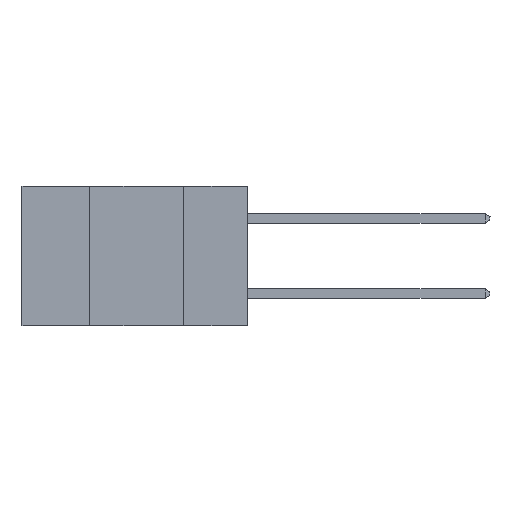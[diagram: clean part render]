
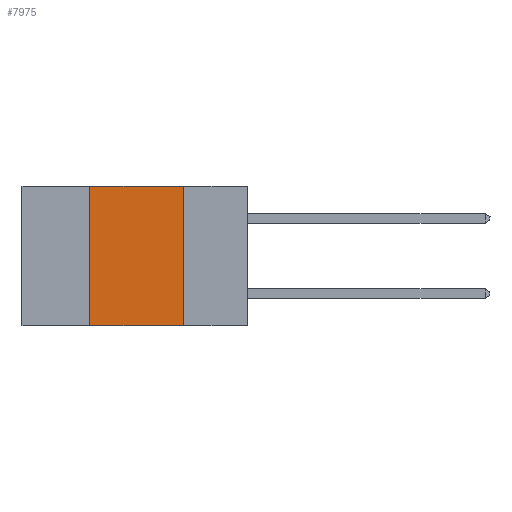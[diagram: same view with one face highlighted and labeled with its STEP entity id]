
A CAD part, left-side view. The second image highlights one B-rep face of the part: STEP entity #7975.
In plain terms, the highlighted planar face has unit normal (-1, 0, 0).
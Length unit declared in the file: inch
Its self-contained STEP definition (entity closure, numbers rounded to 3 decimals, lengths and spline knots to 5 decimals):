
#816 = DIRECTION ( 'NONE',  ( 0., -1., 0. ) ) ;
#1131 = VECTOR ( 'NONE', #14248, 39.37008 ) ;
#1354 = CARTESIAN_POINT ( 'NONE',  ( 0., 0.17, 0. ) ) ;
#2077 = AXIS2_PLACEMENT_3D ( 'NONE', #14946, #12684, #5671 ) ;
#2091 = PLANE ( 'NONE',  #2077 ) ;
#2705 = CARTESIAN_POINT ( 'NONE',  ( 0., 0.17, 0. ) ) ;
#2757 = DIRECTION ( 'NONE',  ( 0., 0., -1. ) ) ;
#2898 = LINE ( 'NONE', #6655, #14089 ) ;
#4205 = VERTEX_POINT ( 'NONE', #1354 ) ;
#4261 = LINE ( 'NONE', #10693, #1131 ) ;
#5671 = DIRECTION ( 'NONE',  ( 0., 0., -1. ) ) ;
#6041 = EDGE_CURVE ( 'NONE', #4205, #9123, #14986, .T. ) ;
#6506 = VERTEX_POINT ( 'NONE', #11519 ) ;
#6655 = CARTESIAN_POINT ( 'NONE',  ( 0., 0.6, 0. ) ) ;
#6948 = CARTESIAN_POINT ( 'NONE',  ( 0., 0.42, 0. ) ) ;
#7524 = EDGE_LOOP ( 'NONE', ( #14388, #11140, #7563, #8151 ) ) ;
#7563 = ORIENTED_EDGE ( 'NONE', *, *, #14990, .F. ) ;
#7975 = ADVANCED_FACE ( 'NONE', ( #11282 ), #2091, .F. ) ;
#8071 = VERTEX_POINT ( 'NONE', #6948 ) ;
#8151 = ORIENTED_EDGE ( 'NONE', *, *, #9171, .T. ) ;
#9123 = VERTEX_POINT ( 'NONE', #15063 ) ;
#9171 = EDGE_CURVE ( 'NONE', #6506, #9123, #9586, .T. ) ;
#9586 = LINE ( 'NONE', #12583, #11964 ) ;
#10693 = CARTESIAN_POINT ( 'NONE',  ( 0., 0.42, 0. ) ) ;
#11140 = ORIENTED_EDGE ( 'NONE', *, *, #11485, .F. ) ;
#11282 = FACE_OUTER_BOUND ( 'NONE', #7524, .T. ) ;
#11485 = EDGE_CURVE ( 'NONE', #8071, #4205, #2898, .T. ) ;
#11519 = CARTESIAN_POINT ( 'NONE',  ( 0., 0.42, -0.37 ) ) ;
#11964 = VECTOR ( 'NONE', #816, 39.37008 ) ;
#12218 = VECTOR ( 'NONE', #2757, 39.37008 ) ;
#12583 = CARTESIAN_POINT ( 'NONE',  ( 0., 0.6, -0.37 ) ) ;
#12684 = DIRECTION ( 'NONE',  ( 1., 0., 0. ) ) ;
#14089 = VECTOR ( 'NONE', #14856, 39.37008 ) ;
#14248 = DIRECTION ( 'NONE',  ( 0., 0., 1. ) ) ;
#14388 = ORIENTED_EDGE ( 'NONE', *, *, #6041, .F. ) ;
#14856 = DIRECTION ( 'NONE',  ( 0., -1., 0. ) ) ;
#14946 = CARTESIAN_POINT ( 'NONE',  ( 0., 0.6, 0. ) ) ;
#14986 = LINE ( 'NONE', #2705, #12218 ) ;
#14990 = EDGE_CURVE ( 'NONE', #6506, #8071, #4261, .T. ) ;
#15063 = CARTESIAN_POINT ( 'NONE',  ( 0., 0.17, -0.37 ) ) ;
